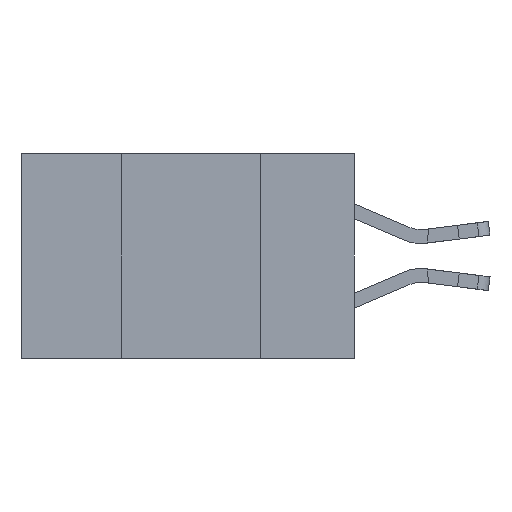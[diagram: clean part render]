
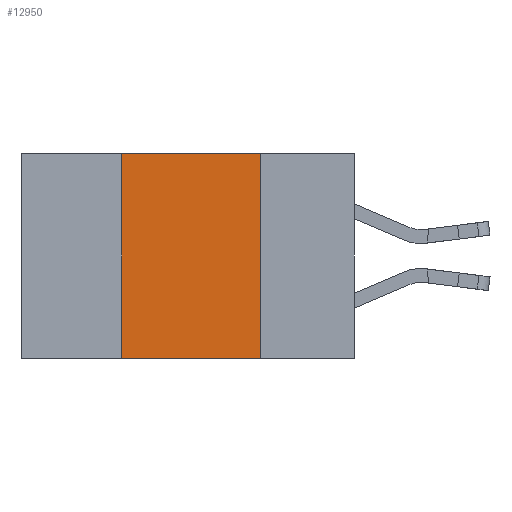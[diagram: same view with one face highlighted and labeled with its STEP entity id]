
A CAD part, left-side view. The second image highlights one B-rep face of the part: STEP entity #12950.
In plain terms, the highlighted planar face has unit normal (-1, 0, 0).
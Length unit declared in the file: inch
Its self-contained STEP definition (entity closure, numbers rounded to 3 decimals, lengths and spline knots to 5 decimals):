
#110 = CARTESIAN_POINT ( 'NONE',  ( 0., 0.17, -0.37 ) ) ;
#980 = VERTEX_POINT ( 'NONE', #110 ) ;
#1741 = ORIENTED_EDGE ( 'NONE', *, *, #5805, .T. ) ;
#2323 = EDGE_LOOP ( 'NONE', ( #5250, #9084, #12744, #1741 ) ) ;
#3068 = FACE_OUTER_BOUND ( 'NONE', #2323, .T. ) ;
#4796 = VECTOR ( 'NONE', #11501, 39.37008 ) ;
#5087 = VECTOR ( 'NONE', #16670, 39.37008 ) ;
#5250 = ORIENTED_EDGE ( 'NONE', *, *, #12106, .F. ) ;
#5805 = EDGE_CURVE ( 'NONE', #17325, #980, #17406, .T. ) ;
#6823 = VECTOR ( 'NONE', #10887, 39.37008 ) ;
#6838 = CARTESIAN_POINT ( 'NONE',  ( 0., 0.42, 0. ) ) ;
#8430 = CARTESIAN_POINT ( 'NONE',  ( 0., 0.42, -0.37 ) ) ;
#9084 = ORIENTED_EDGE ( 'NONE', *, *, #11769, .F. ) ;
#9509 = DIRECTION ( 'NONE',  ( 0., 0., -1. ) ) ;
#10038 = DIRECTION ( 'NONE',  ( 0., 0., -1. ) ) ;
#10245 = EDGE_CURVE ( 'NONE', #17325, #15641, #15823, .T. ) ;
#10380 = VECTOR ( 'NONE', #9509, 39.37008 ) ;
#10865 = CARTESIAN_POINT ( 'NONE',  ( 0., 0.6, -0.37 ) ) ;
#10887 = DIRECTION ( 'NONE',  ( 0., -1., 0. ) ) ;
#11285 = CARTESIAN_POINT ( 'NONE',  ( 0., 0.42, -0.37 ) ) ;
#11501 = DIRECTION ( 'NONE',  ( 0., -1., 0. ) ) ;
#11565 = CARTESIAN_POINT ( 'NONE',  ( 0., 0.6, 0. ) ) ;
#11769 = EDGE_CURVE ( 'NONE', #15641, #12775, #11891, .T. ) ;
#11891 = LINE ( 'NONE', #11565, #4796 ) ;
#12106 = EDGE_CURVE ( 'NONE', #12775, #980, #16758, .T. ) ;
#12178 = CARTESIAN_POINT ( 'NONE',  ( 0., 0.17, 0. ) ) ;
#12744 = ORIENTED_EDGE ( 'NONE', *, *, #10245, .F. ) ;
#12775 = VERTEX_POINT ( 'NONE', #12178 ) ;
#12950 = ADVANCED_FACE ( 'NONE', ( #3068 ), #16759, .F. ) ;
#15582 = AXIS2_PLACEMENT_3D ( 'NONE', #16816, #18132, #10038 ) ;
#15641 = VERTEX_POINT ( 'NONE', #6838 ) ;
#15823 = LINE ( 'NONE', #8430, #5087 ) ;
#16670 = DIRECTION ( 'NONE',  ( 0., 0., 1. ) ) ;
#16758 = LINE ( 'NONE', #17638, #10380 ) ;
#16759 = PLANE ( 'NONE',  #15582 ) ;
#16816 = CARTESIAN_POINT ( 'NONE',  ( 0., 0.6, 0. ) ) ;
#17325 = VERTEX_POINT ( 'NONE', #11285 ) ;
#17406 = LINE ( 'NONE', #10865, #6823 ) ;
#17638 = CARTESIAN_POINT ( 'NONE',  ( 0., 0.17, -0.37 ) ) ;
#18132 = DIRECTION ( 'NONE',  ( 1., 0., 0. ) ) ;
